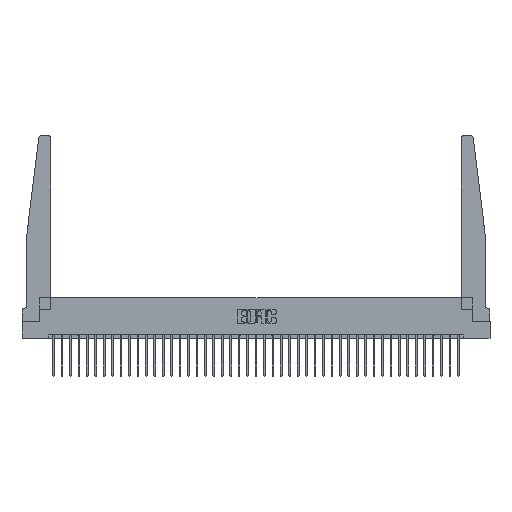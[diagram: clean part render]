
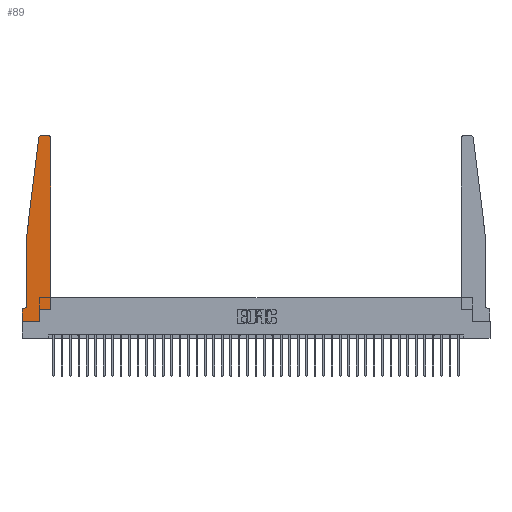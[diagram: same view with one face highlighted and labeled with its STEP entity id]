
A CAD part, top view. The second image highlights one B-rep face of the part: STEP entity #89.
In plain terms, the highlighted planar face has unit normal (0, 0, 1).
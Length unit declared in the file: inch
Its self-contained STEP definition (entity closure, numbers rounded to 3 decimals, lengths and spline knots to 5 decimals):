
#89 = ADVANCED_FACE ( 'NONE', ( #1993 ), #1783, .T. ) ;
#263 = ORIENTED_EDGE ( 'NONE', *, *, #23779, .T. ) ;
#866 = DIRECTION ( 'NONE',  ( -1., 0., 0. ) ) ;
#960 = DIRECTION ( 'NONE',  ( -0.122, -0.992, 0. ) ) ;
#1105 = CARTESIAN_POINT ( 'NONE',  ( 0.425, 2.72, 0.37 ) ) ;
#1447 = DIRECTION ( 'NONE',  ( 0., -1., 0. ) ) ;
#1765 = DIRECTION ( 'NONE',  ( 0., 0., -1. ) ) ;
#1783 = PLANE ( 'NONE',  #15930 ) ;
#1993 = FACE_OUTER_BOUND ( 'NONE', #11038, .T. ) ;
#2607 = VECTOR ( 'NONE', #1447, 39.37008 ) ;
#2625 = LINE ( 'NONE', #30600, #4350 ) ;
#3177 = VERTEX_POINT ( 'NONE', #15991 ) ;
#3611 = VERTEX_POINT ( 'NONE', #4627 ) ;
#3718 = CARTESIAN_POINT ( 'NONE',  ( 0.425, 0.18, 0.37 ) ) ;
#3865 = CARTESIAN_POINT ( 'NONE',  ( 0.425, 0.18, 0.37 ) ) ;
#4341 = EDGE_CURVE ( 'NONE', #11697, #3611, #15072, .T. ) ;
#4350 = VECTOR ( 'NONE', #13989, 39.37008 ) ;
#4627 = CARTESIAN_POINT ( 'NONE',  ( 0.24675, 2.72367, 0.37 ) ) ;
#4986 = CARTESIAN_POINT ( 'NONE',  ( 0.27653, 2.75, 0.37 ) ) ;
#5164 = CARTESIAN_POINT ( 'NONE',  ( 0.395, 2.72, 0.37 ) ) ;
#5261 = VECTOR ( 'NONE', #10142, 39.37008 ) ;
#6178 = VERTEX_POINT ( 'NONE', #6181 ) ;
#6181 = CARTESIAN_POINT ( 'NONE',  ( 0.015, 0.1875, 0.37 ) ) ;
#6481 = VECTOR ( 'NONE', #20691, 39.37008 ) ;
#6902 = CARTESIAN_POINT ( 'NONE',  ( 0.25, 2.75, 0.37 ) ) ;
#7068 = DIRECTION ( 'NONE',  ( -1., 0., 0. ) ) ;
#7357 = CARTESIAN_POINT ( 'NONE',  ( 0.065, 1.25, 0.37 ) ) ;
#7538 = ORIENTED_EDGE ( 'NONE', *, *, #34531, .T. ) ;
#7946 = ORIENTED_EDGE ( 'NONE', *, *, #4341, .T. ) ;
#8412 = LINE ( 'NONE', #3865, #33983 ) ;
#8991 = VECTOR ( 'NONE', #960, 39.37008 ) ;
#9682 = CARTESIAN_POINT ( 'NONE',  ( 0., 0., 0.37 ) ) ;
#9944 = LINE ( 'NONE', #22678, #2607 ) ;
#10087 = ORIENTED_EDGE ( 'NONE', *, *, #33594, .T. ) ;
#10142 = DIRECTION ( 'NONE',  ( 0., 1., 0. ) ) ;
#10207 = DIRECTION ( 'NONE',  ( 1., 0., 0. ) ) ;
#10267 = CARTESIAN_POINT ( 'NONE',  ( 0.425, 0.18, 0.37 ) ) ;
#10297 = AXIS2_PLACEMENT_3D ( 'NONE', #12622, #1765, #7068 ) ;
#10338 = DIRECTION ( 'NONE',  ( 1., 0., 0. ) ) ;
#10439 = CARTESIAN_POINT ( 'NONE',  ( 0.27653, 2.72, 0.37 ) ) ;
#10717 = DIRECTION ( 'NONE',  ( 0., 0., 1. ) ) ;
#11038 = EDGE_LOOP ( 'NONE', ( #34598, #7946, #20531, #16759, #10087, #26325, #29591, #263, #7538, #15790, #24505, #24694 ) ) ;
#11116 = CIRCLE ( 'NONE', #29636, 0.03 ) ;
#11139 = EDGE_CURVE ( 'NONE', #18814, #11990, #13872, .T. ) ;
#11697 = VERTEX_POINT ( 'NONE', #4986 ) ;
#11990 = VERTEX_POINT ( 'NONE', #32183 ) ;
#12139 = DIRECTION ( 'NONE',  ( -1., 0., 0. ) ) ;
#12622 = CARTESIAN_POINT ( 'NONE',  ( 0.015, 0.2375, 0.37 ) ) ;
#13233 = EDGE_CURVE ( 'NONE', #23566, #25631, #9944, .T. ) ;
#13616 = VECTOR ( 'NONE', #866, 39.37008 ) ;
#13872 = LINE ( 'NONE', #9682, #6481 ) ;
#13989 = DIRECTION ( 'NONE',  ( 1., 0., 0. ) ) ;
#14411 = VERTEX_POINT ( 'NONE', #17702 ) ;
#14494 = EDGE_CURVE ( 'NONE', #21640, #3177, #11116, .T. ) ;
#15072 = CIRCLE ( 'NONE', #24649, 0.03 ) ;
#15790 = ORIENTED_EDGE ( 'NONE', *, *, #29412, .T. ) ;
#15830 = EDGE_CURVE ( 'NONE', #3177, #11697, #27068, .T. ) ;
#15930 = AXIS2_PLACEMENT_3D ( 'NONE', #22840, #17242, #31186 ) ;
#15991 = CARTESIAN_POINT ( 'NONE',  ( 0.395, 2.75, 0.37 ) ) ;
#16759 = ORIENTED_EDGE ( 'NONE', *, *, #13233, .T. ) ;
#16944 = LINE ( 'NONE', #26764, #5261 ) ;
#17242 = DIRECTION ( 'NONE',  ( 0., 0., 1. ) ) ;
#17303 = EDGE_CURVE ( 'NONE', #6178, #18814, #20429, .T. ) ;
#17702 = CARTESIAN_POINT ( 'NONE',  ( 0.2605, 0., 0.37 ) ) ;
#18814 = VERTEX_POINT ( 'NONE', #23253 ) ;
#20429 = LINE ( 'NONE', #25793, #23053 ) ;
#20531 = ORIENTED_EDGE ( 'NONE', *, *, #30038, .T. ) ;
#20564 = DIRECTION ( 'NONE',  ( 0., 1., 0. ) ) ;
#20691 = DIRECTION ( 'NONE',  ( 0., -1., 0. ) ) ;
#21030 = CARTESIAN_POINT ( 'NONE',  ( 0.065, 0.2375, 0.37 ) ) ;
#21305 = VERTEX_POINT ( 'NONE', #30095 ) ;
#21640 = VERTEX_POINT ( 'NONE', #1105 ) ;
#22678 = CARTESIAN_POINT ( 'NONE',  ( 0.065, 1.25, 0.37 ) ) ;
#22840 = CARTESIAN_POINT ( 'NONE',  ( 0., 0.1875, 0.37 ) ) ;
#23053 = VECTOR ( 'NONE', #12139, 39.37008 ) ;
#23253 = CARTESIAN_POINT ( 'NONE',  ( 0., 0.1875, 0.37 ) ) ;
#23566 = VERTEX_POINT ( 'NONE', #7357 ) ;
#23779 = EDGE_CURVE ( 'NONE', #11990, #14411, #2625, .T. ) ;
#24505 = ORIENTED_EDGE ( 'NONE', *, *, #28095, .T. ) ;
#24649 = AXIS2_PLACEMENT_3D ( 'NONE', #10439, #32253, #10207 ) ;
#24694 = ORIENTED_EDGE ( 'NONE', *, *, #14494, .T. ) ;
#25057 = LINE ( 'NONE', #31599, #8991 ) ;
#25631 = VERTEX_POINT ( 'NONE', #21030 ) ;
#25793 = CARTESIAN_POINT ( 'NONE',  ( 0.065, 0.1875, 0.37 ) ) ;
#26325 = ORIENTED_EDGE ( 'NONE', *, *, #17303, .T. ) ;
#26564 = VECTOR ( 'NONE', #10338, 39.37008 ) ;
#26764 = CARTESIAN_POINT ( 'NONE',  ( 0.2605, 0.18, 0.37 ) ) ;
#27068 = LINE ( 'NONE', #6902, #13616 ) ;
#28095 = EDGE_CURVE ( 'NONE', #34601, #21640, #8412, .T. ) ;
#29412 = EDGE_CURVE ( 'NONE', #21305, #34601, #33889, .T. ) ;
#29591 = ORIENTED_EDGE ( 'NONE', *, *, #11139, .T. ) ;
#29636 = AXIS2_PLACEMENT_3D ( 'NONE', #5164, #10717, #30104 ) ;
#30038 = EDGE_CURVE ( 'NONE', #3611, #23566, #25057, .T. ) ;
#30095 = CARTESIAN_POINT ( 'NONE',  ( 0.2605, 0.18, 0.37 ) ) ;
#30104 = DIRECTION ( 'NONE',  ( 1., 0., 0. ) ) ;
#30600 = CARTESIAN_POINT ( 'NONE',  ( 0., 0., 0.37 ) ) ;
#31186 = DIRECTION ( 'NONE',  ( 1., 0., 0. ) ) ;
#31599 = CARTESIAN_POINT ( 'NONE',  ( 0.065, 1.25, 0.37 ) ) ;
#32183 = CARTESIAN_POINT ( 'NONE',  ( 0., 0., 0.37 ) ) ;
#32253 = DIRECTION ( 'NONE',  ( 0., 0., 1. ) ) ;
#33412 = CIRCLE ( 'NONE', #10297, 0.05 ) ;
#33594 = EDGE_CURVE ( 'NONE', #25631, #6178, #33412, .T. ) ;
#33889 = LINE ( 'NONE', #3718, #26564 ) ;
#33983 = VECTOR ( 'NONE', #20564, 39.37008 ) ;
#34531 = EDGE_CURVE ( 'NONE', #14411, #21305, #16944, .T. ) ;
#34598 = ORIENTED_EDGE ( 'NONE', *, *, #15830, .T. ) ;
#34601 = VERTEX_POINT ( 'NONE', #10267 ) ;
